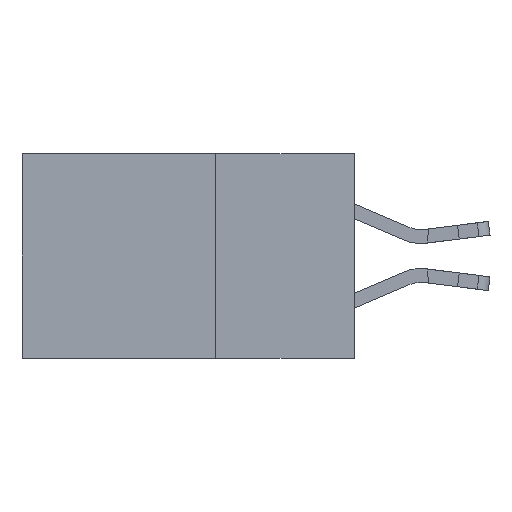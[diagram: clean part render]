
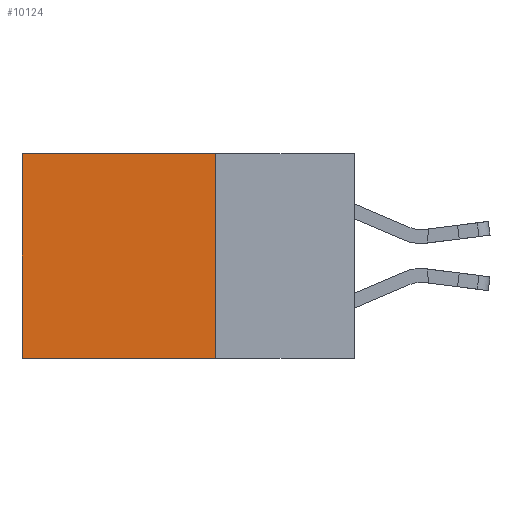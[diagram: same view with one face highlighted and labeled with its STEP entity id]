
A CAD part, left-side view. The second image highlights one B-rep face of the part: STEP entity #10124.
In plain terms, the highlighted planar face has unit normal (-1, 0, 0).
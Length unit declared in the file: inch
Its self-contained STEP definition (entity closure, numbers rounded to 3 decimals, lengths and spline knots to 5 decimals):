
#731 = CARTESIAN_POINT ( 'NONE',  ( 0.298, 0.25, -0.37 ) ) ;
#1084 = CARTESIAN_POINT ( 'NONE',  ( 0.298, 0.25, 0. ) ) ;
#1499 = VECTOR ( 'NONE', #13233, 39.37008 ) ;
#2710 = EDGE_CURVE ( 'NONE', #12768, #16774, #17673, .T. ) ;
#4747 = FACE_OUTER_BOUND ( 'NONE', #21186, .T. ) ;
#4910 = EDGE_CURVE ( 'NONE', #17641, #6706, #15602, .T. ) ;
#5986 = ORIENTED_EDGE ( 'NONE', *, *, #12514, .T. ) ;
#6706 = VERTEX_POINT ( 'NONE', #11996 ) ;
#8002 = CARTESIAN_POINT ( 'NONE',  ( 0.298, 0.6, -0.37 ) ) ;
#8239 = DIRECTION ( 'NONE',  ( 0., 0., -1. ) ) ;
#9456 = ORIENTED_EDGE ( 'NONE', *, *, #18657, .F. ) ;
#10124 = ADVANCED_FACE ( 'NONE', ( #4747 ), #21332, .F. ) ;
#10669 = VECTOR ( 'NONE', #16692, 39.37008 ) ;
#11135 = DIRECTION ( 'NONE',  ( 0., 1., 0. ) ) ;
#11595 = VECTOR ( 'NONE', #8239, 39.37008 ) ;
#11956 = LINE ( 'NONE', #16932, #1499 ) ;
#11996 = CARTESIAN_POINT ( 'NONE',  ( 0.298, 0.6, 0. ) ) ;
#12281 = DIRECTION ( 'NONE',  ( 0., 0., -1. ) ) ;
#12514 = EDGE_CURVE ( 'NONE', #6706, #16774, #11956, .T. ) ;
#12768 = VERTEX_POINT ( 'NONE', #21155 ) ;
#13233 = DIRECTION ( 'NONE',  ( 0., 0., -1. ) ) ;
#15123 = ORIENTED_EDGE ( 'NONE', *, *, #2710, .F. ) ;
#15379 = VECTOR ( 'NONE', #11135, 39.37008 ) ;
#15602 = LINE ( 'NONE', #16816, #10669 ) ;
#16692 = DIRECTION ( 'NONE',  ( 0., 1., 0. ) ) ;
#16774 = VERTEX_POINT ( 'NONE', #8002 ) ;
#16816 = CARTESIAN_POINT ( 'NONE',  ( 0.298, 0.25, 0. ) ) ;
#16932 = CARTESIAN_POINT ( 'NONE',  ( 0.298, 0.6, 0. ) ) ;
#17641 = VERTEX_POINT ( 'NONE', #23680 ) ;
#17673 = LINE ( 'NONE', #731, #15379 ) ;
#18657 = EDGE_CURVE ( 'NONE', #17641, #12768, #20739, .T. ) ;
#19280 = CARTESIAN_POINT ( 'NONE',  ( 0.298, 0.25, 0. ) ) ;
#19922 = ORIENTED_EDGE ( 'NONE', *, *, #4910, .T. ) ;
#19980 = AXIS2_PLACEMENT_3D ( 'NONE', #1084, #23121, #12281 ) ;
#20739 = LINE ( 'NONE', #19280, #11595 ) ;
#21155 = CARTESIAN_POINT ( 'NONE',  ( 0.298, 0.25, -0.37 ) ) ;
#21186 = EDGE_LOOP ( 'NONE', ( #5986, #15123, #9456, #19922 ) ) ;
#21332 = PLANE ( 'NONE',  #19980 ) ;
#23121 = DIRECTION ( 'NONE',  ( 1., 0., 0. ) ) ;
#23680 = CARTESIAN_POINT ( 'NONE',  ( 0.298, 0.25, 0. ) ) ;
